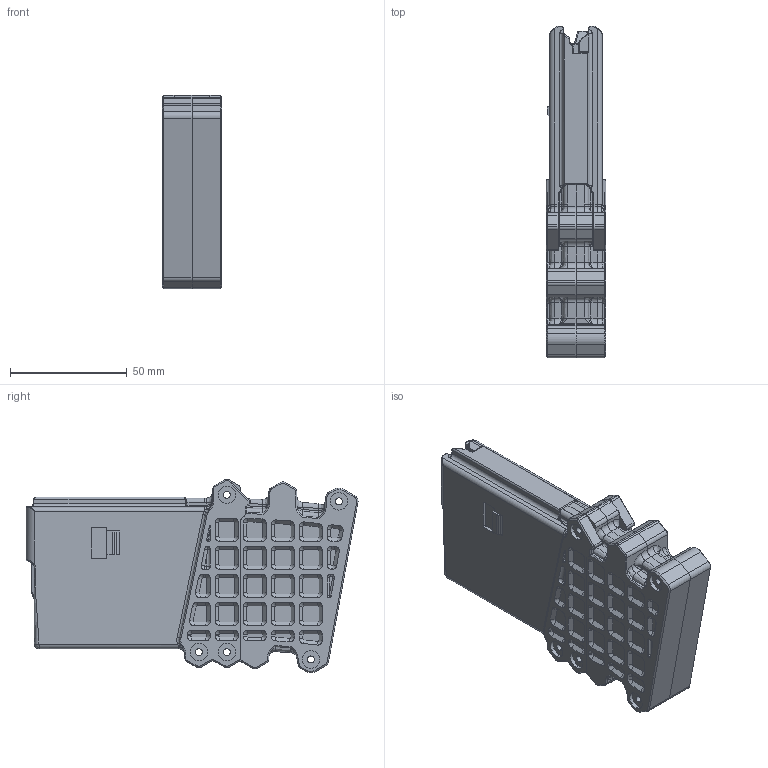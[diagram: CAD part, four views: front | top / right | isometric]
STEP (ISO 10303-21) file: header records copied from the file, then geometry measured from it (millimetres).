
FILE_DESCRIPTION (( 'STEP AP214' ), '1' );
FILE_NAME ('Twenty Round Magazine.STEP', '2021-05-01T22:57:23', ( '' ), ( '' ), 'SwSTEP 2.0', 'SolidWorks 2020', '' );
FILE_SCHEMA (( 'AUTOMOTIVE_DESIGN' ));
Length unit declared in the file: millimetre
Products named in the file (5): Twenty Round Mag Body Bottom Right; Twenty Round Mag Body Bottom Left; Mag Body Top; Mag Follower; Twenty Round Magazine
Assembly tree (4 placements, depth 2):
  Twenty Round Magazine
    Mag Body Top
    Mag Follower
    Twenty Round Mag Body Bottom Left
    Twenty Round Mag Body Bottom Right
Bounding box: 25.5 x 142.2 x 82.82 mm (x, y, z)
Volume: 86840.1 mm3; surface area: 62174.3 mm2
Topology: 4 solids, 4 shells, 2277 faces, 5851 edges, 3566 vertices
Faces by surface type: plane 679, cylinder 649, bspline 502, cone 278, torus 140, sphere 29
Entity records: 86233 total; most frequent: CARTESIAN_POINT 34914, ORIENTED_EDGE 11502, DIRECTION 9736, EDGE_CURVE 5751, AXIS2_PLACEMENT_3D 3583, VERTEX_POINT 3557, LINE 2570, VECTOR 2570
